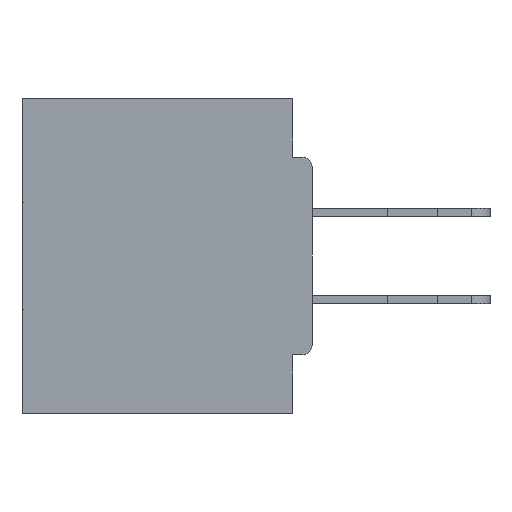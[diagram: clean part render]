
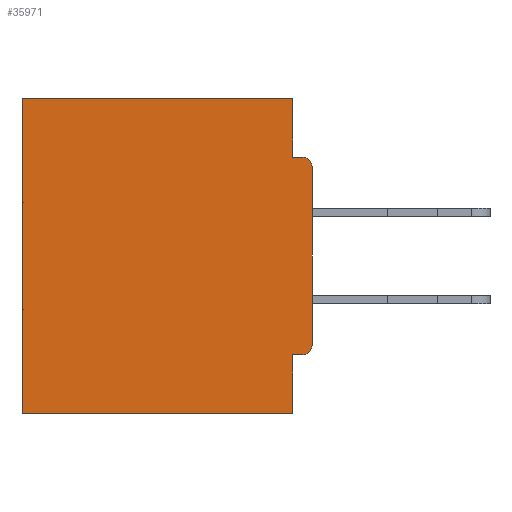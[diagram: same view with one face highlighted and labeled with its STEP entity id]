
A CAD part, left-side view. The second image highlights one B-rep face of the part: STEP entity #35971.
In plain terms, the highlighted planar face has unit normal (-1, 0, 0).
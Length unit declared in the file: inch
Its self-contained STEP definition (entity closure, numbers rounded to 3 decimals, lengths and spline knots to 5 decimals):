
#752 = DIRECTION ( 'NONE',  ( 0., 0., -1. ) ) ;
#2304 = LINE ( 'NONE', #25311, #8415 ) ;
#2584 = VECTOR ( 'NONE', #33050, 39.37008 ) ;
#2880 = CARTESIAN_POINT ( 'NONE',  ( 0.298, 0., 0. ) ) ;
#3816 = EDGE_CURVE ( 'NONE', #10627, #8701, #42218, .T. ) ;
#3895 = VERTEX_POINT ( 'NONE', #4884 ) ;
#3965 = EDGE_CURVE ( 'NONE', #8938, #5038, #2304, .T. ) ;
#4455 = CARTESIAN_POINT ( 'NONE',  ( 0.298, 0.031, -0.4065 ) ) ;
#4884 = CARTESIAN_POINT ( 'NONE',  ( 0.298, 0., -0.1085 ) ) ;
#5038 = VERTEX_POINT ( 'NONE', #35202 ) ;
#5351 = AXIS2_PLACEMENT_3D ( 'NONE', #26382, #19509, #19365 ) ;
#7741 = EDGE_CURVE ( 'NONE', #3895, #11255, #23525, .T. ) ;
#8415 = VECTOR ( 'NONE', #19139, 39.37008 ) ;
#8701 = VERTEX_POINT ( 'NONE', #21937 ) ;
#8727 = ORIENTED_EDGE ( 'NONE', *, *, #24643, .T. ) ;
#8938 = VERTEX_POINT ( 'NONE', #29140 ) ;
#9281 = DIRECTION ( 'NONE',  ( 0., 1., 0. ) ) ;
#10627 = VERTEX_POINT ( 'NONE', #19778 ) ;
#10699 = LINE ( 'NONE', #14658, #17338 ) ;
#11255 = VERTEX_POINT ( 'NONE', #22890 ) ;
#11810 = ORIENTED_EDGE ( 'NONE', *, *, #7741, .F. ) ;
#12540 = CARTESIAN_POINT ( 'NONE',  ( 0.298, 0.46, 0. ) ) ;
#13148 = CARTESIAN_POINT ( 'NONE',  ( 0.298, 0.015, -0.4065 ) ) ;
#13817 = VERTEX_POINT ( 'NONE', #4455 ) ;
#14216 = DIRECTION ( 'NONE',  ( -1., 0., 0. ) ) ;
#14538 = VECTOR ( 'NONE', #9281, 39.37008 ) ;
#14658 = CARTESIAN_POINT ( 'NONE',  ( 0.298, 0.031, -0.5 ) ) ;
#14814 = ORIENTED_EDGE ( 'NONE', *, *, #34537, .T. ) ;
#15500 = ORIENTED_EDGE ( 'NONE', *, *, #18889, .T. ) ;
#15768 = LINE ( 'NONE', #12540, #41351 ) ;
#16534 = ORIENTED_EDGE ( 'NONE', *, *, #3965, .F. ) ;
#17021 = DIRECTION ( 'NONE',  ( 1., 0., 0. ) ) ;
#17338 = VECTOR ( 'NONE', #33844, 39.37008 ) ;
#17402 = CARTESIAN_POINT ( 'NONE',  ( 0.298, 0., -0.4065 ) ) ;
#18106 = ORIENTED_EDGE ( 'NONE', *, *, #38043, .F. ) ;
#18889 = EDGE_CURVE ( 'NONE', #22465, #11255, #40732, .T. ) ;
#19139 = DIRECTION ( 'NONE',  ( 0., 1., 0. ) ) ;
#19365 = DIRECTION ( 'NONE',  ( 0., 0., -1. ) ) ;
#19509 = DIRECTION ( 'NONE',  ( -1., 0., 0. ) ) ;
#19778 = CARTESIAN_POINT ( 'NONE',  ( 0.298, 0.031, -0.0935 ) ) ;
#20097 = FACE_OUTER_BOUND ( 'NONE', #24691, .T. ) ;
#20664 = DIRECTION ( 'NONE',  ( 0., -1., 0. ) ) ;
#21937 = CARTESIAN_POINT ( 'NONE',  ( 0.298, 0.015, -0.0935 ) ) ;
#22080 = VERTEX_POINT ( 'NONE', #30835 ) ;
#22176 = LINE ( 'NONE', #2880, #14538 ) ;
#22465 = VERTEX_POINT ( 'NONE', #13148 ) ;
#22726 = ORIENTED_EDGE ( 'NONE', *, *, #3816, .F. ) ;
#22798 = VECTOR ( 'NONE', #20664, 39.37008 ) ;
#22890 = CARTESIAN_POINT ( 'NONE',  ( 0.298, 0., -0.3915 ) ) ;
#23525 = LINE ( 'NONE', #39794, #37757 ) ;
#24108 = VERTEX_POINT ( 'NONE', #30263 ) ;
#24462 = EDGE_CURVE ( 'NONE', #22465, #13817, #40389, .T. ) ;
#24643 = EDGE_CURVE ( 'NONE', #3895, #8701, #36785, .T. ) ;
#24691 = EDGE_LOOP ( 'NONE', ( #8727, #22726, #40978, #14814, #34936, #16534, #18106, #27882, #15500, #11810 ) ) ;
#25016 = EDGE_CURVE ( 'NONE', #24108, #5038, #15768, .T. ) ;
#25311 = CARTESIAN_POINT ( 'NONE',  ( 0.298, 0., -0.5 ) ) ;
#26382 = CARTESIAN_POINT ( 'NONE',  ( 0.298, 0.015, -0.1085 ) ) ;
#27172 = LINE ( 'NONE', #32911, #2584 ) ;
#27882 = ORIENTED_EDGE ( 'NONE', *, *, #24462, .F. ) ;
#29140 = CARTESIAN_POINT ( 'NONE',  ( 0.298, 0.031, -0.5 ) ) ;
#30052 = PLANE ( 'NONE',  #31183 ) ;
#30263 = CARTESIAN_POINT ( 'NONE',  ( 0.298, 0.46, 0. ) ) ;
#30294 = EDGE_CURVE ( 'NONE', #22080, #10627, #27172, .T. ) ;
#30835 = CARTESIAN_POINT ( 'NONE',  ( 0.298, 0.031, 0. ) ) ;
#31183 = AXIS2_PLACEMENT_3D ( 'NONE', #36585, #17021, #752 ) ;
#32911 = CARTESIAN_POINT ( 'NONE',  ( 0.298, 0.031, -0.5 ) ) ;
#33050 = DIRECTION ( 'NONE',  ( 0., 0., -1. ) ) ;
#33817 = CARTESIAN_POINT ( 'NONE',  ( 0.298, 0.015, -0.3915 ) ) ;
#33844 = DIRECTION ( 'NONE',  ( 0., 0., -1. ) ) ;
#34283 = VECTOR ( 'NONE', #40268, 39.37008 ) ;
#34537 = EDGE_CURVE ( 'NONE', #22080, #24108, #22176, .T. ) ;
#34936 = ORIENTED_EDGE ( 'NONE', *, *, #25016, .T. ) ;
#35202 = CARTESIAN_POINT ( 'NONE',  ( 0.298, 0.46, -0.5 ) ) ;
#35971 = ADVANCED_FACE ( 'NONE', ( #20097 ), #30052, .F. ) ;
#36585 = CARTESIAN_POINT ( 'NONE',  ( 0.298, 0., 0. ) ) ;
#36648 = DIRECTION ( 'NONE',  ( 0., 0., -1. ) ) ;
#36725 = AXIS2_PLACEMENT_3D ( 'NONE', #33817, #14216, #40348 ) ;
#36785 = CIRCLE ( 'NONE', #5351, 0.015 ) ;
#36938 = CARTESIAN_POINT ( 'NONE',  ( 0.298, 0., -0.0935 ) ) ;
#37757 = VECTOR ( 'NONE', #36648, 39.37008 ) ;
#38043 = EDGE_CURVE ( 'NONE', #13817, #8938, #10699, .T. ) ;
#39794 = CARTESIAN_POINT ( 'NONE',  ( 0.298, 0., 0. ) ) ;
#40268 = DIRECTION ( 'NONE',  ( 0., 1., 0. ) ) ;
#40348 = DIRECTION ( 'NONE',  ( 0., 0., -1. ) ) ;
#40389 = LINE ( 'NONE', #17402, #34283 ) ;
#40732 = CIRCLE ( 'NONE', #36725, 0.015 ) ;
#40978 = ORIENTED_EDGE ( 'NONE', *, *, #30294, .F. ) ;
#41351 = VECTOR ( 'NONE', #41989, 39.37008 ) ;
#41989 = DIRECTION ( 'NONE',  ( 0., 0., -1. ) ) ;
#42218 = LINE ( 'NONE', #36938, #22798 ) ;
